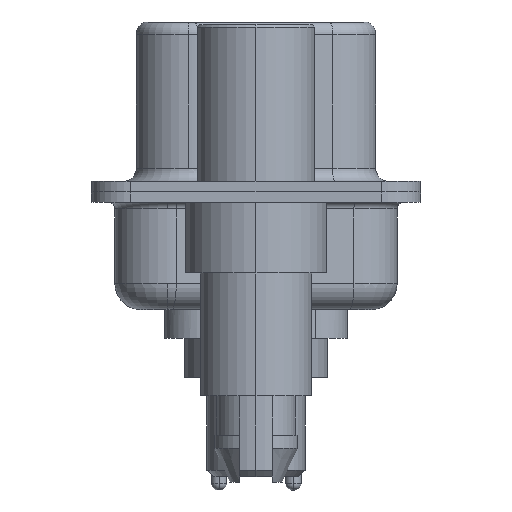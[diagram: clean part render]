
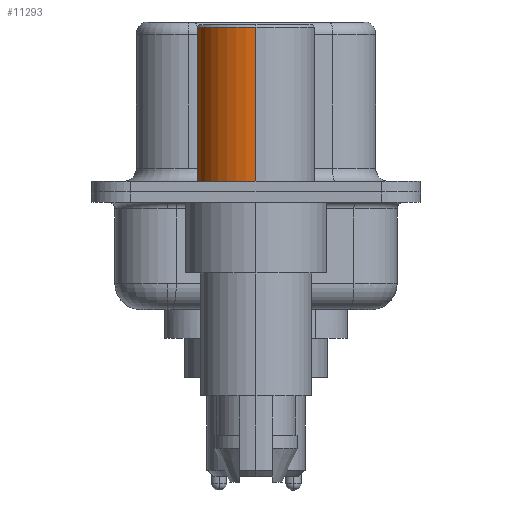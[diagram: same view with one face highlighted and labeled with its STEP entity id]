
A CAD part, left-side view. The second image highlights one B-rep face of the part: STEP entity #11293.
In plain terms, the highlighted cylindrical face has radius 2.25 mm (diameter 4.5 mm), a partial arc.
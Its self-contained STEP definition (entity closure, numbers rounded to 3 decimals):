
#1049 = DIRECTION ( 'NONE',  ( 1., 0., 0. ) ) ;
#1676 = CARTESIAN_POINT ( 'NONE',  ( 2.25, 0., 0.581 ) ) ;
#1698 = LINE ( 'NONE', #1676, #10124 ) ;
#1829 = VERTEX_POINT ( 'NONE', #18244 ) ;
#2362 = DIRECTION ( 'NONE',  ( 0., 0., 1. ) ) ;
#2463 = DIRECTION ( 'NONE',  ( 0., 0., 1. ) ) ;
#2766 = VERTEX_POINT ( 'NONE', #10442 ) ;
#5195 = CARTESIAN_POINT ( 'NONE',  ( 0., 0., 0.4 ) ) ;
#5682 = DIRECTION ( 'NONE',  ( 1., 0., 0. ) ) ;
#6907 = DIRECTION ( 'NONE',  ( 1., 0., 0. ) ) ;
#7260 = CARTESIAN_POINT ( 'NONE',  ( -2.25, 0., 0.4 ) ) ;
#7901 = ORIENTED_EDGE ( 'NONE', *, *, #20846, .F. ) ;
#8381 = DIRECTION ( 'NONE',  ( 0., 0., 1. ) ) ;
#8550 = CYLINDRICAL_SURFACE ( 'NONE', #19296, 2.25 ) ;
#9620 = VECTOR ( 'NONE', #2463, 1000. ) ;
#10124 = VECTOR ( 'NONE', #8381, 1000. ) ;
#10442 = CARTESIAN_POINT ( 'NONE',  ( -2.25, 0., 6.3 ) ) ;
#10674 = EDGE_CURVE ( 'NONE', #21641, #2766, #14038, .T. ) ;
#10893 = CARTESIAN_POINT ( 'NONE',  ( -2.25, 0., 0.581 ) ) ;
#11086 = EDGE_CURVE ( 'NONE', #16439, #21641, #20677, .T. ) ;
#11158 = DIRECTION ( 'NONE',  ( 0., 0., 1. ) ) ;
#11293 = ADVANCED_FACE ( 'NONE', ( #17497 ), #8550, .T. ) ;
#11781 = ORIENTED_EDGE ( 'NONE', *, *, #10674, .T. ) ;
#12718 = ORIENTED_EDGE ( 'NONE', *, *, #11086, .T. ) ;
#12726 = EDGE_CURVE ( 'NONE', #1829, #2766, #17700, .T. ) ;
#12881 = AXIS2_PLACEMENT_3D ( 'NONE', #5195, #17012, #6907 ) ;
#12900 = CARTESIAN_POINT ( 'NONE',  ( 2.25, 0., 0.4 ) ) ;
#14038 = LINE ( 'NONE', #10893, #9620 ) ;
#15849 = CARTESIAN_POINT ( 'NONE',  ( 0., 0., 0.581 ) ) ;
#16439 = VERTEX_POINT ( 'NONE', #12900 ) ;
#17012 = DIRECTION ( 'NONE',  ( 0., 0., 1. ) ) ;
#17497 = FACE_OUTER_BOUND ( 'NONE', #19012, .T. ) ;
#17700 = CIRCLE ( 'NONE', #21327, 2.25 ) ;
#18244 = CARTESIAN_POINT ( 'NONE',  ( 2.25, 0., 6.3 ) ) ;
#19012 = EDGE_LOOP ( 'NONE', ( #12718, #11781, #20337, #7901 ) ) ;
#19296 = AXIS2_PLACEMENT_3D ( 'NONE', #15849, #2362, #5682 ) ;
#20337 = ORIENTED_EDGE ( 'NONE', *, *, #12726, .F. ) ;
#20677 = CIRCLE ( 'NONE', #12881, 2.25 ) ;
#20846 = EDGE_CURVE ( 'NONE', #16439, #1829, #1698, .T. ) ;
#21258 = CARTESIAN_POINT ( 'NONE',  ( 0., 0., 6.3 ) ) ;
#21327 = AXIS2_PLACEMENT_3D ( 'NONE', #21258, #11158, #1049 ) ;
#21641 = VERTEX_POINT ( 'NONE', #7260 ) ;
